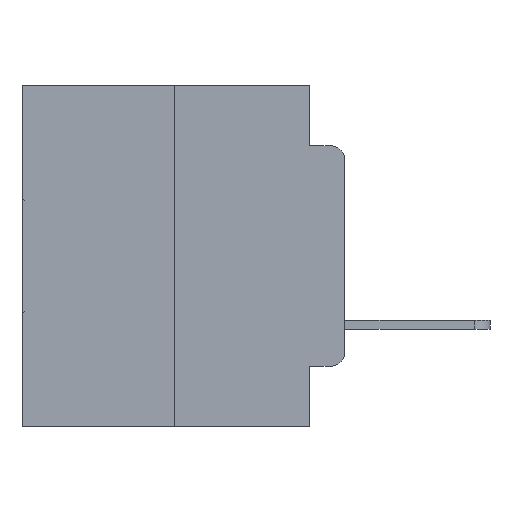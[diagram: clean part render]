
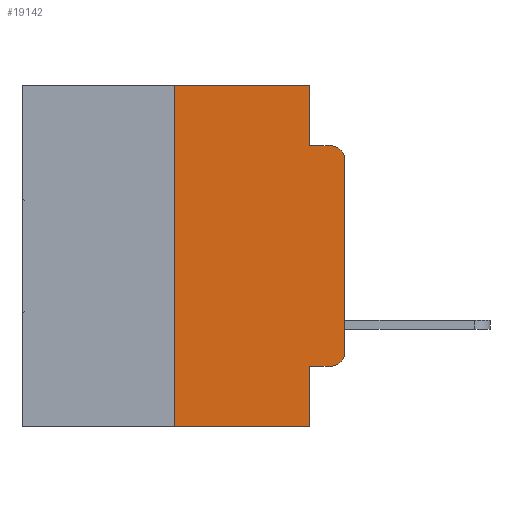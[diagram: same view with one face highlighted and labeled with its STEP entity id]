
A CAD part, left-side view. The second image highlights one B-rep face of the part: STEP entity #19142.
In plain terms, the highlighted planar face has unit normal (-1, 0, 0).
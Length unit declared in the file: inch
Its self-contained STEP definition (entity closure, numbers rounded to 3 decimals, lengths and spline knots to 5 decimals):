
#67 = EDGE_CURVE ( 'NONE', #9201, #13922, #4580, .T. ) ;
#269 = DIRECTION ( 'NONE',  ( 0., 0., -1. ) ) ;
#1166 = VECTOR ( 'NONE', #9075, 39.37008 ) ;
#1214 = CARTESIAN_POINT ( 'NONE',  ( 0., 0.051, 0. ) ) ;
#1269 = DIRECTION ( 'NONE',  ( 0., 0., -1. ) ) ;
#1283 = DIRECTION ( 'NONE',  ( 0., 0., -1. ) ) ;
#1897 = DIRECTION ( 'NONE',  ( 0., 0., -1. ) ) ;
#3834 = VECTOR ( 'NONE', #1269, 39.37008 ) ;
#4580 = LINE ( 'NONE', #10759, #3834 ) ;
#4882 = CARTESIAN_POINT ( 'NONE',  ( 0., 0.051, -0.5 ) ) ;
#5012 = VECTOR ( 'NONE', #23990, 39.37008 ) ;
#5584 = CARTESIAN_POINT ( 'NONE',  ( 0., 0.473, 0. ) ) ;
#5604 = ORIENTED_EDGE ( 'NONE', *, *, #21418, .T. ) ;
#5708 = EDGE_LOOP ( 'NONE', ( #12097, #6506, #24714, #6994, #23792, #19300, #5604, #25754, #17932, #25904 ) ) ;
#6331 = CARTESIAN_POINT ( 'NONE',  ( 0., 0., -0.3915 ) ) ;
#6391 = VECTOR ( 'NONE', #14211, 39.37008 ) ;
#6506 = ORIENTED_EDGE ( 'NONE', *, *, #9443, .T. ) ;
#6638 = DIRECTION ( 'NONE',  ( 0., -1., 0. ) ) ;
#6737 = CARTESIAN_POINT ( 'NONE',  ( 0., 0.473, -0.5 ) ) ;
#6994 = ORIENTED_EDGE ( 'NONE', *, *, #67, .F. ) ;
#7002 = VECTOR ( 'NONE', #6638, 39.37008 ) ;
#7592 = CARTESIAN_POINT ( 'NONE',  ( 0., 0.25, -0.5 ) ) ;
#8293 = CIRCLE ( 'NONE', #8658, 0.02 ) ;
#8428 = FACE_OUTER_BOUND ( 'NONE', #5708, .T. ) ;
#8430 = VECTOR ( 'NONE', #19386, 39.37008 ) ;
#8658 = AXIS2_PLACEMENT_3D ( 'NONE', #26116, #12511, #28289 ) ;
#9075 = DIRECTION ( 'NONE',  ( 0., -1., 0. ) ) ;
#9201 = VERTEX_POINT ( 'NONE', #1214 ) ;
#9443 = EDGE_CURVE ( 'NONE', #19592, #23495, #26122, .T. ) ;
#10759 = CARTESIAN_POINT ( 'NONE',  ( 0., 0.051, 0. ) ) ;
#11182 = VERTEX_POINT ( 'NONE', #18060 ) ;
#11549 = VERTEX_POINT ( 'NONE', #21715 ) ;
#11921 = CARTESIAN_POINT ( 'NONE',  ( 0., 0., 0. ) ) ;
#12097 = ORIENTED_EDGE ( 'NONE', *, *, #29063, .T. ) ;
#12511 = DIRECTION ( 'NONE',  ( -1., 0., 0. ) ) ;
#12568 = CARTESIAN_POINT ( 'NONE',  ( 0., 0.051, -0.0885 ) ) ;
#12591 = VERTEX_POINT ( 'NONE', #6331 ) ;
#12644 = EDGE_CURVE ( 'NONE', #16072, #9201, #19123, .T. ) ;
#13070 = CARTESIAN_POINT ( 'NONE',  ( 0., 0.25, 0. ) ) ;
#13071 = EDGE_CURVE ( 'NONE', #13922, #23495, #20526, .T. ) ;
#13166 = AXIS2_PLACEMENT_3D ( 'NONE', #5584, #15262, #1283 ) ;
#13239 = VECTOR ( 'NONE', #1897, 39.37008 ) ;
#13708 = CARTESIAN_POINT ( 'NONE',  ( 0., 0.051, -0.0885 ) ) ;
#13803 = VECTOR ( 'NONE', #24418, 39.37008 ) ;
#13922 = VERTEX_POINT ( 'NONE', #13708 ) ;
#14045 = VERTEX_POINT ( 'NONE', #4882 ) ;
#14211 = DIRECTION ( 'NONE',  ( 0., 0., 1. ) ) ;
#14296 = DIRECTION ( 'NONE',  ( -1., 0., 0. ) ) ;
#14499 = CARTESIAN_POINT ( 'NONE',  ( 0., 0.02, -0.0885 ) ) ;
#14507 = LINE ( 'NONE', #13070, #13803 ) ;
#15262 = DIRECTION ( 'NONE',  ( 1., 0., 0. ) ) ;
#16072 = VERTEX_POINT ( 'NONE', #19391 ) ;
#17932 = ORIENTED_EDGE ( 'NONE', *, *, #26867, .T. ) ;
#18060 = CARTESIAN_POINT ( 'NONE',  ( 0., 0.051, -0.4115 ) ) ;
#19123 = LINE ( 'NONE', #22616, #7002 ) ;
#19142 = ADVANCED_FACE ( 'NONE', ( #8428 ), #28723, .F. ) ;
#19157 = EDGE_CURVE ( 'NONE', #25225, #16072, #14507, .T. ) ;
#19251 = LINE ( 'NONE', #22580, #13239 ) ;
#19300 = ORIENTED_EDGE ( 'NONE', *, *, #19157, .F. ) ;
#19386 = DIRECTION ( 'NONE',  ( 0., -1., 0. ) ) ;
#19391 = CARTESIAN_POINT ( 'NONE',  ( 0., 0.25, 0. ) ) ;
#19592 = VERTEX_POINT ( 'NONE', #28235 ) ;
#20526 = LINE ( 'NONE', #12568, #8430 ) ;
#21418 = EDGE_CURVE ( 'NONE', #25225, #14045, #24305, .T. ) ;
#21676 = CARTESIAN_POINT ( 'NONE',  ( 0., 0.051, -0.4115 ) ) ;
#21715 = CARTESIAN_POINT ( 'NONE',  ( 0., 0.02, -0.4115 ) ) ;
#22041 = EDGE_CURVE ( 'NONE', #11182, #14045, #19251, .T. ) ;
#22580 = CARTESIAN_POINT ( 'NONE',  ( 0., 0.051, 0. ) ) ;
#22616 = CARTESIAN_POINT ( 'NONE',  ( 0., 0.473, 0. ) ) ;
#23327 = LINE ( 'NONE', #21676, #5012 ) ;
#23495 = VERTEX_POINT ( 'NONE', #14499 ) ;
#23792 = ORIENTED_EDGE ( 'NONE', *, *, #12644, .F. ) ;
#23990 = DIRECTION ( 'NONE',  ( 0., -1., 0. ) ) ;
#24305 = LINE ( 'NONE', #6737, #1166 ) ;
#24418 = DIRECTION ( 'NONE',  ( 0., 0., 1. ) ) ;
#24640 = LINE ( 'NONE', #11921, #6391 ) ;
#24714 = ORIENTED_EDGE ( 'NONE', *, *, #13071, .F. ) ;
#24795 = AXIS2_PLACEMENT_3D ( 'NONE', #27820, #14296, #269 ) ;
#25225 = VERTEX_POINT ( 'NONE', #7592 ) ;
#25754 = ORIENTED_EDGE ( 'NONE', *, *, #22041, .F. ) ;
#25904 = ORIENTED_EDGE ( 'NONE', *, *, #27412, .T. ) ;
#26116 = CARTESIAN_POINT ( 'NONE',  ( 0., 0.02, -0.3915 ) ) ;
#26122 = CIRCLE ( 'NONE', #24795, 0.02 ) ;
#26867 = EDGE_CURVE ( 'NONE', #11182, #11549, #23327, .T. ) ;
#27412 = EDGE_CURVE ( 'NONE', #11549, #12591, #8293, .T. ) ;
#27820 = CARTESIAN_POINT ( 'NONE',  ( 0., 0.02, -0.1085 ) ) ;
#28235 = CARTESIAN_POINT ( 'NONE',  ( 0., 0., -0.1085 ) ) ;
#28289 = DIRECTION ( 'NONE',  ( 0., 0., -1. ) ) ;
#28723 = PLANE ( 'NONE',  #13166 ) ;
#29063 = EDGE_CURVE ( 'NONE', #12591, #19592, #24640, .T. ) ;
